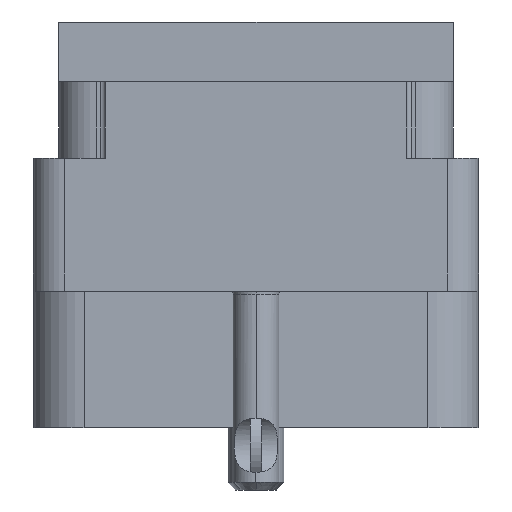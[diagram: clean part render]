
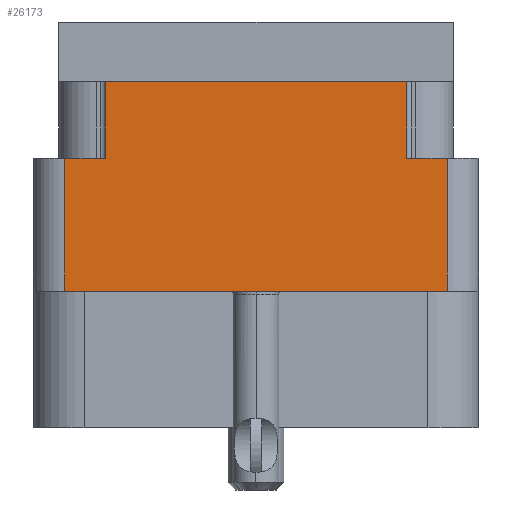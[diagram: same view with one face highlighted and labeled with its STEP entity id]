
A CAD part, left-side view. The second image highlights one B-rep face of the part: STEP entity #26173.
In plain terms, the highlighted planar face has unit normal (-1, 0, 0).
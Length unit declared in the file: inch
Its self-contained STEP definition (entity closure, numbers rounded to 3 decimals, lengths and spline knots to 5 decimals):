
#273 = CARTESIAN_POINT ( 'NONE',  ( -1., 0.376, -0.529 ) ) ;
#635 = DIRECTION ( 'NONE',  ( 0., 0., 1. ) ) ;
#663 = LINE ( 'NONE', #33694, #27101 ) ;
#2101 = VECTOR ( 'NONE', #32461, 39.37008 ) ;
#2639 = LINE ( 'NONE', #22835, #2101 ) ;
#2682 = VERTEX_POINT ( 'NONE', #16096 ) ;
#2764 = EDGE_CURVE ( 'NONE', #17304, #16866, #6586, .T. ) ;
#3869 = EDGE_CURVE ( 'NONE', #2682, #7015, #23765, .T. ) ;
#4672 = ORIENTED_EDGE ( 'NONE', *, *, #20642, .T. ) ;
#6586 = LINE ( 'NONE', #19066, #17776 ) ;
#7015 = VERTEX_POINT ( 'NONE', #8847 ) ;
#7020 = ORIENTED_EDGE ( 'NONE', *, *, #35491, .T. ) ;
#8236 = CARTESIAN_POINT ( 'NONE',  ( -1., 0.296, -0.117 ) ) ;
#8327 = ORIENTED_EDGE ( 'NONE', *, *, #2764, .F. ) ;
#8372 = VERTEX_POINT ( 'NONE', #38185 ) ;
#8847 = CARTESIAN_POINT ( 'NONE',  ( -1., 0.296, -0.268 ) ) ;
#8896 = CARTESIAN_POINT ( 'NONE',  ( -1., -0.296, -0.117 ) ) ;
#9047 = DIRECTION ( 'NONE',  ( 0., 0., 1. ) ) ;
#11536 = EDGE_CURVE ( 'NONE', #24371, #2682, #15350, .T. ) ;
#11866 = CARTESIAN_POINT ( 'NONE',  ( -1., -0.296, -0.268 ) ) ;
#12043 = LINE ( 'NONE', #11866, #16625 ) ;
#14761 = DIRECTION ( 'NONE',  ( 0., -1., 0. ) ) ;
#15106 = ORIENTED_EDGE ( 'NONE', *, *, #26418, .T. ) ;
#15165 = VECTOR ( 'NONE', #14761, 39.37008 ) ;
#15350 = LINE ( 'NONE', #20732, #33579 ) ;
#15644 = LINE ( 'NONE', #38649, #18688 ) ;
#16096 = CARTESIAN_POINT ( 'NONE',  ( -1., 0.376, -0.268 ) ) ;
#16625 = VECTOR ( 'NONE', #9047, 39.37008 ) ;
#16855 = DIRECTION ( 'NONE',  ( -1., 0., 0. ) ) ;
#16866 = VERTEX_POINT ( 'NONE', #8896 ) ;
#17304 = VERTEX_POINT ( 'NONE', #8236 ) ;
#17585 = DIRECTION ( 'NONE',  ( 0., -1., 0. ) ) ;
#17776 = VECTOR ( 'NONE', #22291, 39.37008 ) ;
#18648 = EDGE_CURVE ( 'NONE', #31881, #8372, #663, .T. ) ;
#18688 = VECTOR ( 'NONE', #29039, 39.37008 ) ;
#19066 = CARTESIAN_POINT ( 'NONE',  ( -1., 0.438, -0.117 ) ) ;
#20319 = VERTEX_POINT ( 'NONE', #36947 ) ;
#20642 = EDGE_CURVE ( 'NONE', #24371, #20319, #2639, .T. ) ;
#20732 = CARTESIAN_POINT ( 'NONE',  ( -1., 0.376, -0.798 ) ) ;
#22291 = DIRECTION ( 'NONE',  ( 0., -1., 0. ) ) ;
#22835 = CARTESIAN_POINT ( 'NONE',  ( -1., 0., -0.529 ) ) ;
#23765 = LINE ( 'NONE', #28348, #15165 ) ;
#23933 = ORIENTED_EDGE ( 'NONE', *, *, #3869, .F. ) ;
#24371 = VERTEX_POINT ( 'NONE', #273 ) ;
#26173 = ADVANCED_FACE ( 'NONE', ( #39690 ), #26756, .T. ) ;
#26418 = EDGE_CURVE ( 'NONE', #20319, #8372, #27029, .T. ) ;
#26756 = PLANE ( 'NONE',  #40764 ) ;
#27029 = LINE ( 'NONE', #28002, #37164 ) ;
#27101 = VECTOR ( 'NONE', #17585, 39.37008 ) ;
#28002 = CARTESIAN_POINT ( 'NONE',  ( -1., -0.376, -0.798 ) ) ;
#28348 = CARTESIAN_POINT ( 'NONE',  ( -1., 0.438, -0.268 ) ) ;
#29039 = DIRECTION ( 'NONE',  ( 0., 0., 1. ) ) ;
#29081 = ORIENTED_EDGE ( 'NONE', *, *, #30928, .F. ) ;
#30013 = ORIENTED_EDGE ( 'NONE', *, *, #11536, .F. ) ;
#30928 = EDGE_CURVE ( 'NONE', #7015, #17304, #15644, .T. ) ;
#31881 = VERTEX_POINT ( 'NONE', #34637 ) ;
#32461 = DIRECTION ( 'NONE',  ( 0., -1., 0. ) ) ;
#33579 = VECTOR ( 'NONE', #40501, 39.37008 ) ;
#33694 = CARTESIAN_POINT ( 'NONE',  ( -1., -0.296, -0.268 ) ) ;
#34637 = CARTESIAN_POINT ( 'NONE',  ( -1., -0.296, -0.268 ) ) ;
#34806 = EDGE_LOOP ( 'NONE', ( #30013, #4672, #15106, #35602, #7020, #8327, #29081, #23933 ) ) ;
#35361 = DIRECTION ( 'NONE',  ( 0., 0., 1. ) ) ;
#35491 = EDGE_CURVE ( 'NONE', #31881, #16866, #12043, .T. ) ;
#35602 = ORIENTED_EDGE ( 'NONE', *, *, #18648, .F. ) ;
#36220 = CARTESIAN_POINT ( 'NONE',  ( -1., -0.376, -0.798 ) ) ;
#36947 = CARTESIAN_POINT ( 'NONE',  ( -1., -0.376, -0.529 ) ) ;
#37164 = VECTOR ( 'NONE', #35361, 39.37008 ) ;
#38185 = CARTESIAN_POINT ( 'NONE',  ( -1., -0.376, -0.268 ) ) ;
#38649 = CARTESIAN_POINT ( 'NONE',  ( -1., 0.296, -0.268 ) ) ;
#39690 = FACE_OUTER_BOUND ( 'NONE', #34806, .T. ) ;
#40501 = DIRECTION ( 'NONE',  ( 0., 0., 1. ) ) ;
#40764 = AXIS2_PLACEMENT_3D ( 'NONE', #36220, #16855, #635 ) ;
